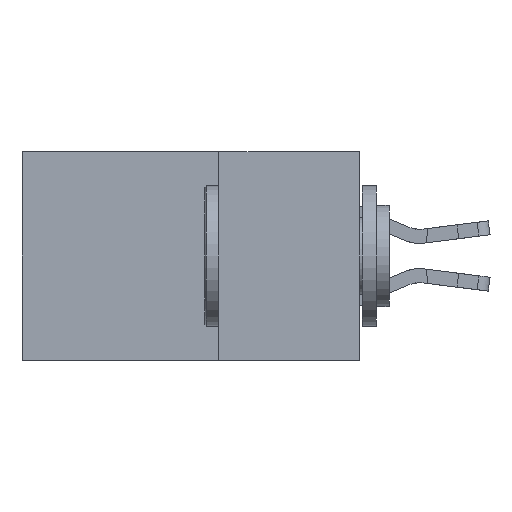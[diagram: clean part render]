
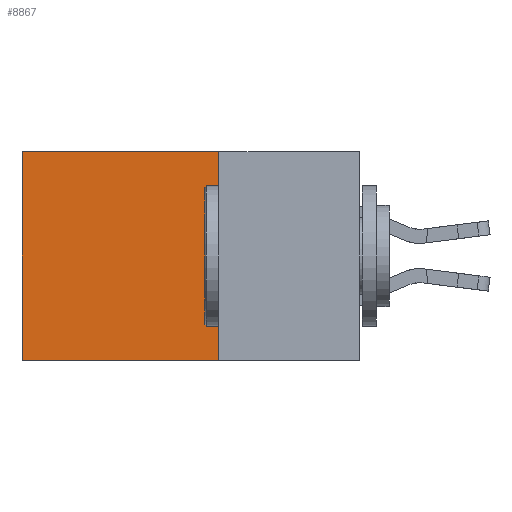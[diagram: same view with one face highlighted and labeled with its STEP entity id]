
A CAD part, left-side view. The second image highlights one B-rep face of the part: STEP entity #8867.
In plain terms, the highlighted planar face has unit normal (-1, 0, 0).
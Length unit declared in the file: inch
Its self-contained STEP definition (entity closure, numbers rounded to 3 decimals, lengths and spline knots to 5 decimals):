
#707 = ORIENTED_EDGE ( 'NONE', *, *, #8414, .T. ) ;
#1635 = ORIENTED_EDGE ( 'NONE', *, *, #3791, .F. ) ;
#1877 = CARTESIAN_POINT ( 'NONE',  ( 0.2875, 0.6, -0.37 ) ) ;
#2087 = EDGE_LOOP ( 'NONE', ( #9739, #4413, #1635, #707 ) ) ;
#2126 = PLANE ( 'NONE',  #9836 ) ;
#3035 = FACE_OUTER_BOUND ( 'NONE', #2087, .T. ) ;
#3791 = EDGE_CURVE ( 'NONE', #9327, #8874, #12136, .T. ) ;
#4004 = DIRECTION ( 'NONE',  ( 0., 0., -1. ) ) ;
#4413 = ORIENTED_EDGE ( 'NONE', *, *, #9840, .F. ) ;
#5110 = CARTESIAN_POINT ( 'NONE',  ( 0.2875, 0.25, 0. ) ) ;
#5454 = VECTOR ( 'NONE', #8515, 39.37008 ) ;
#5577 = VECTOR ( 'NONE', #4004, 39.37008 ) ;
#5661 = CARTESIAN_POINT ( 'NONE',  ( 0.2875, 0.25, 0. ) ) ;
#5968 = CARTESIAN_POINT ( 'NONE',  ( 0.2875, 0.25, 0. ) ) ;
#6170 = CARTESIAN_POINT ( 'NONE',  ( 0.2875, 0.6, 0. ) ) ;
#6272 = DIRECTION ( 'NONE',  ( 0., 1., 0. ) ) ;
#7355 = DIRECTION ( 'NONE',  ( 0., 0., -1. ) ) ;
#7565 = VERTEX_POINT ( 'NONE', #6170 ) ;
#7677 = DIRECTION ( 'NONE',  ( 0., 1., 0. ) ) ;
#8414 = EDGE_CURVE ( 'NONE', #9327, #7565, #13353, .T. ) ;
#8515 = DIRECTION ( 'NONE',  ( 0., 0., -1. ) ) ;
#8604 = CARTESIAN_POINT ( 'NONE',  ( 0.2875, 0.25, -0.37 ) ) ;
#8867 = ADVANCED_FACE ( 'NONE', ( #3035 ), #2126, .F. ) ;
#8874 = VERTEX_POINT ( 'NONE', #8604 ) ;
#9049 = LINE ( 'NONE', #11315, #11945 ) ;
#9327 = VERTEX_POINT ( 'NONE', #5661 ) ;
#9600 = VERTEX_POINT ( 'NONE', #1877 ) ;
#9739 = ORIENTED_EDGE ( 'NONE', *, *, #11185, .T. ) ;
#9836 = AXIS2_PLACEMENT_3D ( 'NONE', #9837, #14799, #7355 ) ;
#9837 = CARTESIAN_POINT ( 'NONE',  ( 0.2875, 0.25, 0. ) ) ;
#9840 = EDGE_CURVE ( 'NONE', #8874, #9600, #9049, .T. ) ;
#11185 = EDGE_CURVE ( 'NONE', #7565, #9600, #15515, .T. ) ;
#11315 = CARTESIAN_POINT ( 'NONE',  ( 0.2875, 0.25, -0.37 ) ) ;
#11945 = VECTOR ( 'NONE', #6272, 39.37008 ) ;
#12136 = LINE ( 'NONE', #5968, #5454 ) ;
#12842 = CARTESIAN_POINT ( 'NONE',  ( 0.2875, 0.6, 0. ) ) ;
#12954 = VECTOR ( 'NONE', #7677, 39.37008 ) ;
#13353 = LINE ( 'NONE', #5110, #12954 ) ;
#14799 = DIRECTION ( 'NONE',  ( 1., 0., 0. ) ) ;
#15515 = LINE ( 'NONE', #12842, #5577 ) ;
